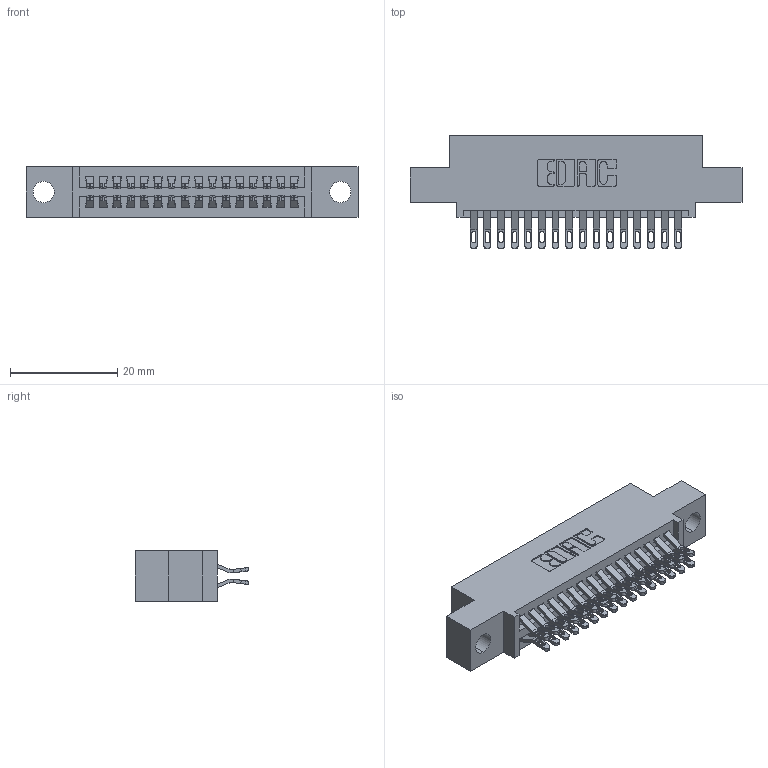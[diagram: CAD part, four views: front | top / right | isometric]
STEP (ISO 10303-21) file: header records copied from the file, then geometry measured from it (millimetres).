
FILE_DESCRIPTION (( 'STEP AP203' ), '1' );
FILE_NAME ('395-032-555-504.STEP', '2021-06-16T20:33:19', ( '' ), ( '' ), 'SwSTEP 2.0', 'SolidWorks 2020', '' );
FILE_SCHEMA (( 'CONFIG_CONTROL_DESIGN' ));
Length unit declared in the file: inch
Products named in the file (3): 345 Part_0.110 Offset - 0.156 Dia-TI; 345-292-001_555 Tail; 395-032-555-504
Assembly tree (33 placements, depth 2):
  395-032-555-504
    345 Part_0.110 Offset - 0.156 Dia-TI
    345-292-001_555 Tail  x32
Bounding box: 61.85 x 21.13 x 9.4 mm (x, y, z)
Volume: 5680.2 mm3; surface area: 8160 mm2
Topology: 33 solids, 33 shells, 1936 faces, 6053 edges, 4034 vertices
Faces by surface type: plane 1090, cylinder 846
Entity records: 16931 total; most frequent: CARTESIAN_POINT 2904, ORIENTED_EDGE 2806, DIRECTION 2559, EDGE_CURVE 1403, VECTOR 1187, LINE 1187, VERTEX_POINT 934, AXIS2_PLACEMENT_3D 686
